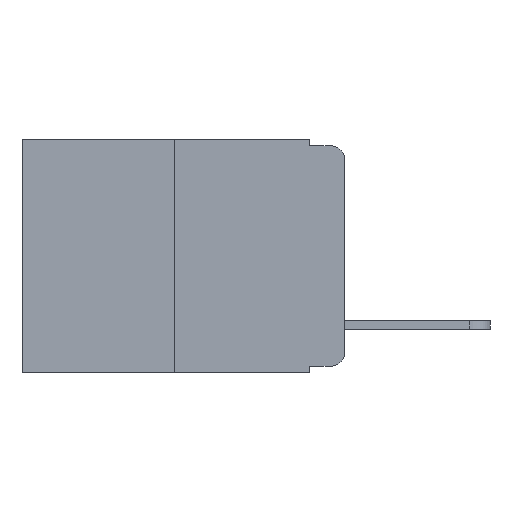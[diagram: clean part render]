
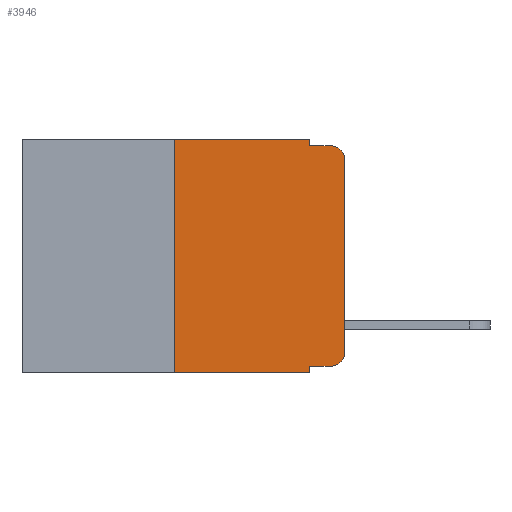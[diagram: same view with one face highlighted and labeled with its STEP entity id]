
A CAD part, left-side view. The second image highlights one B-rep face of the part: STEP entity #3946.
In plain terms, the highlighted planar face has unit normal (-1, 0, 0).
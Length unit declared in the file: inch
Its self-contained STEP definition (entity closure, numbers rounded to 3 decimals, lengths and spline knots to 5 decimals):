
#156 = AXIS2_PLACEMENT_3D ( 'NONE', #6122, #6059, #6014 ) ;
#635 = CARTESIAN_POINT ( 'NONE',  ( 0., 0.051, -0.01 ) ) ;
#896 = DIRECTION ( 'NONE',  ( 0., 0., 1. ) ) ;
#941 = VERTEX_POINT ( 'NONE', #14368 ) ;
#977 = CARTESIAN_POINT ( 'NONE',  ( 0., 0.25, 0. ) ) ;
#1457 = CARTESIAN_POINT ( 'NONE',  ( 0., 0., 0. ) ) ;
#1533 = LINE ( 'NONE', #19274, #14011 ) ;
#1800 = VECTOR ( 'NONE', #19346, 39.37008 ) ;
#2906 = CARTESIAN_POINT ( 'NONE',  ( 0., 0.051, 0. ) ) ;
#3011 = VERTEX_POINT ( 'NONE', #7718 ) ;
#3039 = EDGE_CURVE ( 'NONE', #15640, #16287, #13907, .T. ) ;
#3087 = FACE_OUTER_BOUND ( 'NONE', #9190, .T. ) ;
#3468 = CARTESIAN_POINT ( 'NONE',  ( 0., 0.02, -0.333 ) ) ;
#3946 = ADVANCED_FACE ( 'NONE', ( #3087 ), #17105, .F. ) ;
#4196 = EDGE_CURVE ( 'NONE', #19875, #15640, #17096, .T. ) ;
#4270 = EDGE_CURVE ( 'NONE', #16287, #10667, #8429, .T. ) ;
#4330 = CARTESIAN_POINT ( 'NONE',  ( 0., 0.25, 0. ) ) ;
#4585 = VECTOR ( 'NONE', #896, 39.37008 ) ;
#5175 = CARTESIAN_POINT ( 'NONE',  ( 0., 0.473, 0. ) ) ;
#5479 = CARTESIAN_POINT ( 'NONE',  ( 0., 0., -0.313 ) ) ;
#6014 = DIRECTION ( 'NONE',  ( 0., 0., -1. ) ) ;
#6059 = DIRECTION ( 'NONE',  ( -1., 0., 0. ) ) ;
#6122 = CARTESIAN_POINT ( 'NONE',  ( 0., 0.02, -0.313 ) ) ;
#6266 = VERTEX_POINT ( 'NONE', #3468 ) ;
#6932 = LINE ( 'NONE', #4330, #14890 ) ;
#7144 = DIRECTION ( 'NONE',  ( 0., -1., 0. ) ) ;
#7308 = LINE ( 'NONE', #11750, #18274 ) ;
#7718 = CARTESIAN_POINT ( 'NONE',  ( 0., 0.25, -0.343 ) ) ;
#7838 = EDGE_CURVE ( 'NONE', #3011, #16683, #1533, .T. ) ;
#8429 = LINE ( 'NONE', #19221, #1800 ) ;
#8473 = VERTEX_POINT ( 'NONE', #10807 ) ;
#8681 = LINE ( 'NONE', #2906, #20226 ) ;
#8686 = DIRECTION ( 'NONE',  ( 0., 0., -1. ) ) ;
#8717 = DIRECTION ( 'NONE',  ( -1., 0., 0. ) ) ;
#8821 = CARTESIAN_POINT ( 'NONE',  ( 0., 0.02, -0.03 ) ) ;
#9190 = EDGE_LOOP ( 'NONE', ( #10978, #11410, #11735, #12121, #12725, #13686, #13726, #14311, #14722, #14931 ) ) ;
#9454 = AXIS2_PLACEMENT_3D ( 'NONE', #17659, #13192, #11567 ) ;
#9854 = VECTOR ( 'NONE', #13620, 39.37008 ) ;
#10315 = CARTESIAN_POINT ( 'NONE',  ( 0., 0.051, 0. ) ) ;
#10667 = VERTEX_POINT ( 'NONE', #20821 ) ;
#10807 = CARTESIAN_POINT ( 'NONE',  ( 0., 0.051, -0.333 ) ) ;
#10978 = ORIENTED_EDGE ( 'NONE', *, *, #12224, .T. ) ;
#11200 = EDGE_CURVE ( 'NONE', #941, #10667, #18894, .T. ) ;
#11410 = ORIENTED_EDGE ( 'NONE', *, *, #11200, .T. ) ;
#11567 = DIRECTION ( 'NONE',  ( 0., 0., -1. ) ) ;
#11735 = ORIENTED_EDGE ( 'NONE', *, *, #4270, .F. ) ;
#11750 = CARTESIAN_POINT ( 'NONE',  ( 0., 0.051, -0.333 ) ) ;
#11994 = CIRCLE ( 'NONE', #156, 0.02 ) ;
#12121 = ORIENTED_EDGE ( 'NONE', *, *, #3039, .F. ) ;
#12224 = EDGE_CURVE ( 'NONE', #13631, #941, #16991, .T. ) ;
#12725 = ORIENTED_EDGE ( 'NONE', *, *, #4196, .F. ) ;
#13192 = DIRECTION ( 'NONE',  ( 1., 0., 0. ) ) ;
#13595 = EDGE_CURVE ( 'NONE', #6266, #13631, #11994, .T. ) ;
#13620 = DIRECTION ( 'NONE',  ( 0., 0., -1. ) ) ;
#13631 = VERTEX_POINT ( 'NONE', #5479 ) ;
#13686 = ORIENTED_EDGE ( 'NONE', *, *, #19624, .F. ) ;
#13691 = CARTESIAN_POINT ( 'NONE',  ( 0., 0.051, 0. ) ) ;
#13726 = ORIENTED_EDGE ( 'NONE', *, *, #7838, .T. ) ;
#13907 = LINE ( 'NONE', #13691, #9854 ) ;
#14011 = VECTOR ( 'NONE', #19041, 39.37008 ) ;
#14311 = ORIENTED_EDGE ( 'NONE', *, *, #18697, .F. ) ;
#14368 = CARTESIAN_POINT ( 'NONE',  ( 0., 0., -0.03 ) ) ;
#14546 = DIRECTION ( 'NONE',  ( 0., 0., -1. ) ) ;
#14722 = ORIENTED_EDGE ( 'NONE', *, *, #17663, .T. ) ;
#14890 = VECTOR ( 'NONE', #17281, 39.37008 ) ;
#14931 = ORIENTED_EDGE ( 'NONE', *, *, #13595, .T. ) ;
#15640 = VERTEX_POINT ( 'NONE', #10315 ) ;
#16287 = VERTEX_POINT ( 'NONE', #635 ) ;
#16530 = AXIS2_PLACEMENT_3D ( 'NONE', #8821, #8717, #8686 ) ;
#16683 = VERTEX_POINT ( 'NONE', #20765 ) ;
#16991 = LINE ( 'NONE', #1457, #4585 ) ;
#17096 = LINE ( 'NONE', #5175, #20891 ) ;
#17105 = PLANE ( 'NONE',  #9454 ) ;
#17281 = DIRECTION ( 'NONE',  ( 0., 0., 1. ) ) ;
#17659 = CARTESIAN_POINT ( 'NONE',  ( 0., 0.473, 0. ) ) ;
#17663 = EDGE_CURVE ( 'NONE', #8473, #6266, #7308, .T. ) ;
#18274 = VECTOR ( 'NONE', #19199, 39.37008 ) ;
#18697 = EDGE_CURVE ( 'NONE', #8473, #16683, #8681, .T. ) ;
#18894 = CIRCLE ( 'NONE', #16530, 0.02 ) ;
#19041 = DIRECTION ( 'NONE',  ( 0., -1., 0. ) ) ;
#19199 = DIRECTION ( 'NONE',  ( 0., -1., 0. ) ) ;
#19221 = CARTESIAN_POINT ( 'NONE',  ( 0., 0.051, -0.01 ) ) ;
#19274 = CARTESIAN_POINT ( 'NONE',  ( 0., 0.473, -0.343 ) ) ;
#19346 = DIRECTION ( 'NONE',  ( 0., -1., 0. ) ) ;
#19624 = EDGE_CURVE ( 'NONE', #3011, #19875, #6932, .T. ) ;
#19875 = VERTEX_POINT ( 'NONE', #977 ) ;
#20226 = VECTOR ( 'NONE', #14546, 39.37008 ) ;
#20765 = CARTESIAN_POINT ( 'NONE',  ( 0., 0.051, -0.343 ) ) ;
#20821 = CARTESIAN_POINT ( 'NONE',  ( 0., 0.02, -0.01 ) ) ;
#20891 = VECTOR ( 'NONE', #7144, 39.37008 ) ;
